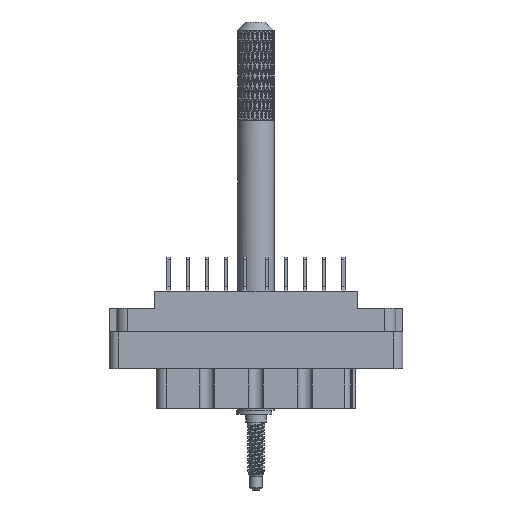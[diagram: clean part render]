
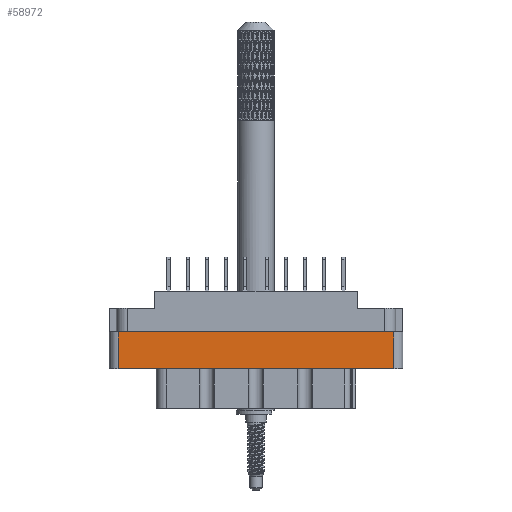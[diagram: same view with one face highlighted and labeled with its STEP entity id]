
A CAD part, front view. The second image highlights one B-rep face of the part: STEP entity #58972.
In plain terms, the highlighted planar face has unit normal (0, -1, 0).
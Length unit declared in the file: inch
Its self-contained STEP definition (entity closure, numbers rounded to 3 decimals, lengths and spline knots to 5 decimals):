
#524 = LINE ( 'NONE', #10819, #32166 ) ;
#3311 = ORIENTED_EDGE ( 'NONE', *, *, #91038, .F. ) ;
#5302 = VECTOR ( 'NONE', #71127, 39.37008 ) ;
#7395 = VECTOR ( 'NONE', #55176, 39.37008 ) ;
#7546 = CARTESIAN_POINT ( 'NONE',  ( 0.938, -0.438, -0.529 ) ) ;
#9612 = CARTESIAN_POINT ( 'NONE',  ( -0.938, -0.438, -0.277 ) ) ;
#10819 = CARTESIAN_POINT ( 'NONE',  ( 0.938, -0.438, -0.798 ) ) ;
#11204 = LINE ( 'NONE', #78822, #7395 ) ;
#11508 = DIRECTION ( 'NONE',  ( 0., 0., 1. ) ) ;
#11611 = LINE ( 'NONE', #48144, #5302 ) ;
#12936 = ORIENTED_EDGE ( 'NONE', *, *, #56389, .T. ) ;
#17897 = VERTEX_POINT ( 'NONE', #38060 ) ;
#29593 = ORIENTED_EDGE ( 'NONE', *, *, #85322, .T. ) ;
#32166 = VECTOR ( 'NONE', #11508, 39.37008 ) ;
#32509 = CARTESIAN_POINT ( 'NONE',  ( -1., -0.438, -0.798 ) ) ;
#32545 = VERTEX_POINT ( 'NONE', #7546 ) ;
#33071 = ORIENTED_EDGE ( 'NONE', *, *, #58668, .F. ) ;
#38060 = CARTESIAN_POINT ( 'NONE',  ( -0.938, -0.438, -0.529 ) ) ;
#44951 = CARTESIAN_POINT ( 'NONE',  ( -0.938, -0.438, -0.798 ) ) ;
#48144 = CARTESIAN_POINT ( 'NONE',  ( 0., -0.438, -0.277 ) ) ;
#53788 = DIRECTION ( 'NONE',  ( 0., 0., -1. ) ) ;
#55176 = DIRECTION ( 'NONE',  ( -1., 0., 0. ) ) ;
#56389 = EDGE_CURVE ( 'NONE', #32545, #104023, #524, .T. ) ;
#58668 = EDGE_CURVE ( 'NONE', #100315, #104023, #11611, .T. ) ;
#58794 = VECTOR ( 'NONE', #53788, 39.37008 ) ;
#58972 = ADVANCED_FACE ( 'NONE', ( #62182 ), #64988, .T. ) ;
#62182 = FACE_OUTER_BOUND ( 'NONE', #89717, .T. ) ;
#64988 = PLANE ( 'NONE',  #90786 ) ;
#66404 = LINE ( 'NONE', #44951, #58794 ) ;
#71127 = DIRECTION ( 'NONE',  ( 1., 0., 0. ) ) ;
#71720 = DIRECTION ( 'NONE',  ( 0., -1., 0. ) ) ;
#78822 = CARTESIAN_POINT ( 'NONE',  ( 0., -0.438, -0.529 ) ) ;
#81496 = CARTESIAN_POINT ( 'NONE',  ( 0.938, -0.438, -0.277 ) ) ;
#85322 = EDGE_CURVE ( 'NONE', #100315, #17897, #66404, .T. ) ;
#88935 = DIRECTION ( 'NONE',  ( 0., 0., -1. ) ) ;
#89717 = EDGE_LOOP ( 'NONE', ( #33071, #29593, #3311, #12936 ) ) ;
#90786 = AXIS2_PLACEMENT_3D ( 'NONE', #32509, #71720, #88935 ) ;
#91038 = EDGE_CURVE ( 'NONE', #32545, #17897, #11204, .T. ) ;
#100315 = VERTEX_POINT ( 'NONE', #9612 ) ;
#104023 = VERTEX_POINT ( 'NONE', #81496 ) ;
